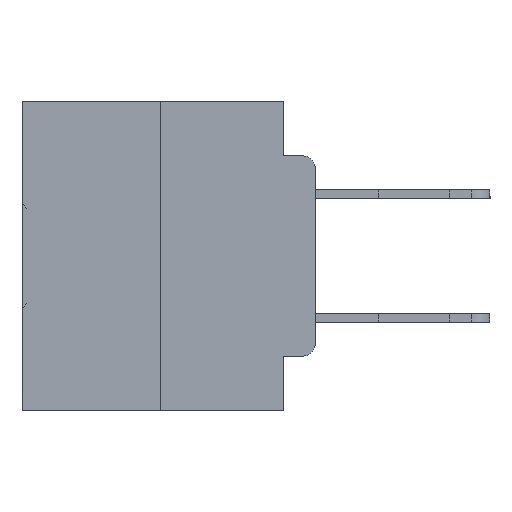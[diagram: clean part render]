
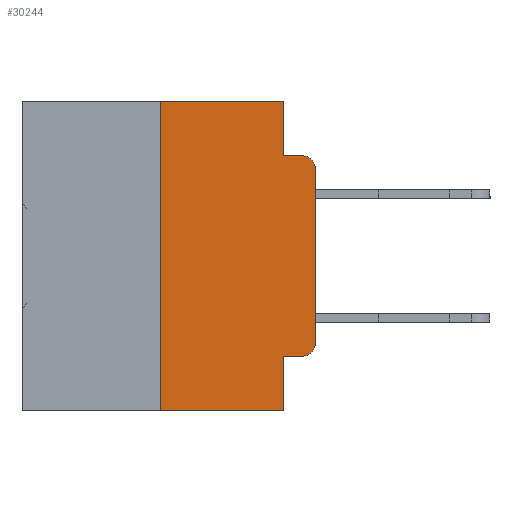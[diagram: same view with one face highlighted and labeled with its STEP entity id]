
A CAD part, left-side view. The second image highlights one B-rep face of the part: STEP entity #30244.
In plain terms, the highlighted planar face has unit normal (-1, 0, 0).
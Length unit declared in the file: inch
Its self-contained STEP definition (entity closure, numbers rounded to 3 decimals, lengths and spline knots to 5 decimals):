
#569 = ORIENTED_EDGE ( 'NONE', *, *, #12220, .T. ) ;
#654 = LINE ( 'NONE', #31590, #6749 ) ;
#748 = EDGE_CURVE ( 'NONE', #15488, #27857, #3117, .T. ) ;
#865 = CARTESIAN_POINT ( 'NONE',  ( 0., 0.25, 0. ) ) ;
#1119 = DIRECTION ( 'NONE',  ( 0., 0., -1. ) ) ;
#1140 = CARTESIAN_POINT ( 'NONE',  ( 0., 0.051, -0.0885 ) ) ;
#1241 = DIRECTION ( 'NONE',  ( 0., -1., 0. ) ) ;
#2652 = ORIENTED_EDGE ( 'NONE', *, *, #16617, .T. ) ;
#3117 = LINE ( 'NONE', #6095, #9172 ) ;
#3366 = EDGE_CURVE ( 'NONE', #3865, #7385, #17946, .T. ) ;
#3658 = DIRECTION ( 'NONE',  ( 0., -1., 0. ) ) ;
#3723 = DIRECTION ( 'NONE',  ( 0., -1., 0. ) ) ;
#3865 = VERTEX_POINT ( 'NONE', #18398 ) ;
#5149 = DIRECTION ( 'NONE',  ( -1., 0., 0. ) ) ;
#5648 = DIRECTION ( 'NONE',  ( 1., 0., 0. ) ) ;
#5649 = AXIS2_PLACEMENT_3D ( 'NONE', #20583, #5149, #23160 ) ;
#5872 = CARTESIAN_POINT ( 'NONE',  ( 0., 0.02, -0.1085 ) ) ;
#6095 = CARTESIAN_POINT ( 'NONE',  ( 0., 0.473, 0. ) ) ;
#6140 = VERTEX_POINT ( 'NONE', #6284 ) ;
#6284 = CARTESIAN_POINT ( 'NONE',  ( 0., 0.25, -0.5 ) ) ;
#6478 = CARTESIAN_POINT ( 'NONE',  ( 0., 0.051, -0.5 ) ) ;
#6749 = VECTOR ( 'NONE', #18693, 39.37008 ) ;
#7245 = LINE ( 'NONE', #11487, #27009 ) ;
#7385 = VERTEX_POINT ( 'NONE', #6478 ) ;
#7742 = CARTESIAN_POINT ( 'NONE',  ( 0., 0.051, 0. ) ) ;
#7824 = CARTESIAN_POINT ( 'NONE',  ( 0., 0.051, 0. ) ) ;
#8208 = CARTESIAN_POINT ( 'NONE',  ( 0., 0.02, -0.4115 ) ) ;
#8454 = DIRECTION ( 'NONE',  ( 0., 0., -1. ) ) ;
#8646 = EDGE_CURVE ( 'NONE', #6140, #15488, #25503, .T. ) ;
#9059 = ORIENTED_EDGE ( 'NONE', *, *, #18941, .T. ) ;
#9092 = ORIENTED_EDGE ( 'NONE', *, *, #8646, .F. ) ;
#9172 = VECTOR ( 'NONE', #11110, 39.37008 ) ;
#9669 = VECTOR ( 'NONE', #3658, 39.37008 ) ;
#10302 = ORIENTED_EDGE ( 'NONE', *, *, #3366, .F. ) ;
#10608 = VERTEX_POINT ( 'NONE', #16794 ) ;
#11110 = DIRECTION ( 'NONE',  ( 0., -1., 0. ) ) ;
#11487 = CARTESIAN_POINT ( 'NONE',  ( 0., 0.473, -0.5 ) ) ;
#12220 = EDGE_CURVE ( 'NONE', #19384, #19736, #654, .T. ) ;
#13408 = AXIS2_PLACEMENT_3D ( 'NONE', #28742, #5648, #23646 ) ;
#14052 = VERTEX_POINT ( 'NONE', #8208 ) ;
#14301 = CIRCLE ( 'NONE', #23354, 0.02 ) ;
#15188 = CARTESIAN_POINT ( 'NONE',  ( 0., 0., -0.3915 ) ) ;
#15476 = FACE_OUTER_BOUND ( 'NONE', #23351, .T. ) ;
#15488 = VERTEX_POINT ( 'NONE', #865 ) ;
#15549 = ORIENTED_EDGE ( 'NONE', *, *, #31009, .F. ) ;
#16147 = EDGE_CURVE ( 'NONE', #3865, #14052, #16550, .T. ) ;
#16550 = LINE ( 'NONE', #26795, #9669 ) ;
#16617 = EDGE_CURVE ( 'NONE', #6140, #7385, #7245, .T. ) ;
#16794 = CARTESIAN_POINT ( 'NONE',  ( 0., 0.051, -0.0885 ) ) ;
#17790 = CARTESIAN_POINT ( 'NONE',  ( 0., 0., -0.1085 ) ) ;
#17946 = LINE ( 'NONE', #7742, #25611 ) ;
#18164 = CIRCLE ( 'NONE', #5649, 0.02 ) ;
#18175 = DIRECTION ( 'NONE',  ( 0., 0., -1. ) ) ;
#18398 = CARTESIAN_POINT ( 'NONE',  ( 0., 0.051, -0.4115 ) ) ;
#18524 = VECTOR ( 'NONE', #1241, 39.37008 ) ;
#18693 = DIRECTION ( 'NONE',  ( 0., 0., 1. ) ) ;
#18941 = EDGE_CURVE ( 'NONE', #19736, #29081, #14301, .T. ) ;
#19384 = VERTEX_POINT ( 'NONE', #15188 ) ;
#19467 = LINE ( 'NONE', #29466, #25521 ) ;
#19736 = VERTEX_POINT ( 'NONE', #17790 ) ;
#20583 = CARTESIAN_POINT ( 'NONE',  ( 0., 0.02, -0.3915 ) ) ;
#20799 = ORIENTED_EDGE ( 'NONE', *, *, #22557, .F. ) ;
#21078 = PLANE ( 'NONE',  #13408 ) ;
#21888 = CARTESIAN_POINT ( 'NONE',  ( 0., 0.02, -0.0885 ) ) ;
#22557 = EDGE_CURVE ( 'NONE', #10608, #29081, #32261, .T. ) ;
#23160 = DIRECTION ( 'NONE',  ( 0., 0., -1. ) ) ;
#23351 = EDGE_LOOP ( 'NONE', ( #569, #9059, #20799, #15549, #27276, #9092, #2652, #10302, #28926, #30578 ) ) ;
#23354 = AXIS2_PLACEMENT_3D ( 'NONE', #5872, #23887, #8454 ) ;
#23646 = DIRECTION ( 'NONE',  ( 0., 0., -1. ) ) ;
#23887 = DIRECTION ( 'NONE',  ( -1., 0., 0. ) ) ;
#24677 = VECTOR ( 'NONE', #31738, 39.37008 ) ;
#25503 = LINE ( 'NONE', #26504, #24677 ) ;
#25521 = VECTOR ( 'NONE', #1119, 39.37008 ) ;
#25611 = VECTOR ( 'NONE', #18175, 39.37008 ) ;
#26504 = CARTESIAN_POINT ( 'NONE',  ( 0., 0.25, 0. ) ) ;
#26795 = CARTESIAN_POINT ( 'NONE',  ( 0., 0.051, -0.4115 ) ) ;
#27009 = VECTOR ( 'NONE', #3723, 39.37008 ) ;
#27276 = ORIENTED_EDGE ( 'NONE', *, *, #748, .F. ) ;
#27857 = VERTEX_POINT ( 'NONE', #7824 ) ;
#28742 = CARTESIAN_POINT ( 'NONE',  ( 0., 0.473, 0. ) ) ;
#28847 = EDGE_CURVE ( 'NONE', #14052, #19384, #18164, .T. ) ;
#28926 = ORIENTED_EDGE ( 'NONE', *, *, #16147, .T. ) ;
#29081 = VERTEX_POINT ( 'NONE', #21888 ) ;
#29466 = CARTESIAN_POINT ( 'NONE',  ( 0., 0.051, 0. ) ) ;
#30244 = ADVANCED_FACE ( 'NONE', ( #15476 ), #21078, .F. ) ;
#30578 = ORIENTED_EDGE ( 'NONE', *, *, #28847, .T. ) ;
#31009 = EDGE_CURVE ( 'NONE', #27857, #10608, #19467, .T. ) ;
#31590 = CARTESIAN_POINT ( 'NONE',  ( 0., 0., 0. ) ) ;
#31738 = DIRECTION ( 'NONE',  ( 0., 0., 1. ) ) ;
#32261 = LINE ( 'NONE', #1140, #18524 ) ;
